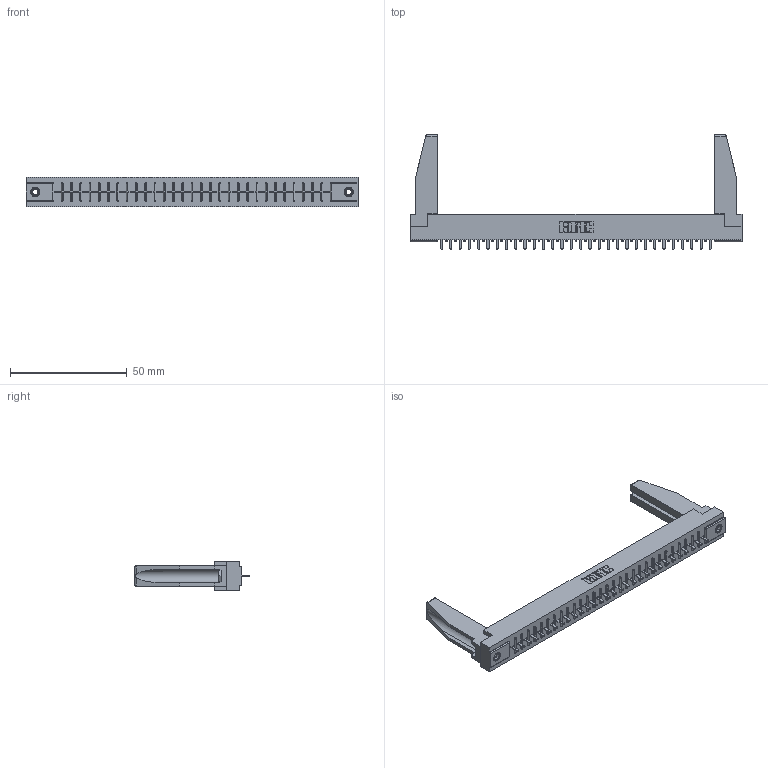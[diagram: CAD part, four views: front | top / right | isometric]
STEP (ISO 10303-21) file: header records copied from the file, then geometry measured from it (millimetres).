
FILE_DESCRIPTION (( 'STEP AP203' ), '1' );
FILE_NAME ('316-030-521-178.STEP', '2018-07-31T03:24:03', ( '' ), ( '' ), 'SwSTEP 2.0', 'SolidWorks 2016', '' );
FILE_SCHEMA (( 'CONFIG_CONTROL_DESIGN' ));
Length unit declared in the file: inch
Products named in the file (5): 307-220-078; 316-030-521-178; 306 Part_.156 Dia; 306-290-001_121; 345-250-001_345-250-001-102
Assembly tree (35 placements, depth 2):
  316-030-521-178
    306 Part_.156 Dia
    306-290-001_121  x30
    345-250-001_345-250-001-102  x2
    307-220-078  x2
Bounding box: 141.88 x 48.92 x 12.7 mm (x, y, z)
Volume: 19541.2 mm3; surface area: 19429.9 mm2
Topology: 35 solids, 35 shells, 2346 faces, 6556 edges, 4200 vertices
Faces by surface type: plane 1562, cylinder 648, sphere 120, cone 12, torus 4
Entity records: 31926 total; most frequent: CARTESIAN_POINT 5359, ORIENTED_EDGE 5270, DIRECTION 5237, EDGE_CURVE 2635, LINE 2057, VECTOR 2057, VERTEX_POINT 1670, AXIS2_PLACEMENT_3D 1590
